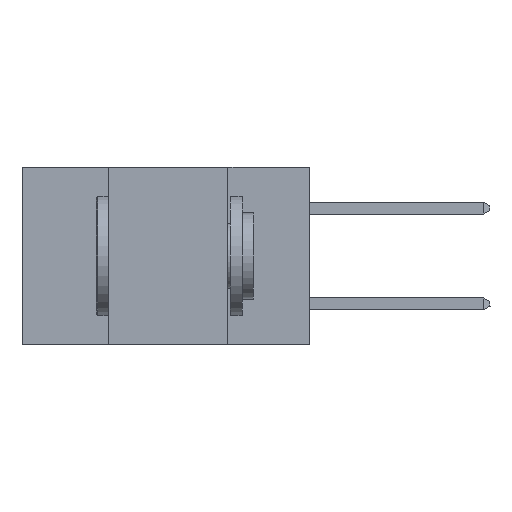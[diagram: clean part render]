
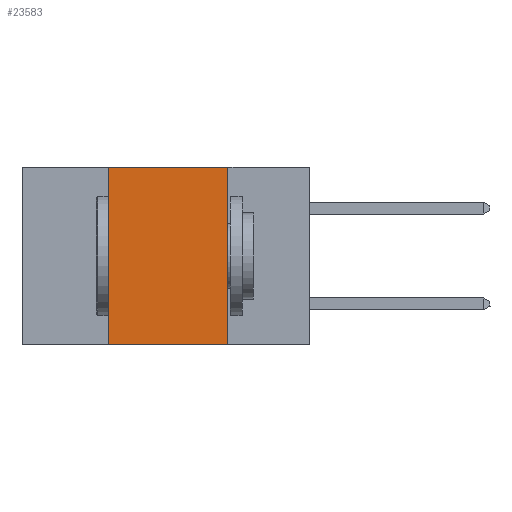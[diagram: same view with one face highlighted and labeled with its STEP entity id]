
A CAD part, left-side view. The second image highlights one B-rep face of the part: STEP entity #23583.
In plain terms, the highlighted planar face has unit normal (-1, 0, 0).
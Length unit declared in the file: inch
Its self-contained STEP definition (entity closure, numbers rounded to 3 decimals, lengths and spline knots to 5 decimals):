
#287 = DIRECTION ( 'NONE',  ( 0., 0., -1. ) ) ;
#386 = EDGE_CURVE ( 'NONE', #21851, #12763, #11255, .T. ) ;
#1092 = CARTESIAN_POINT ( 'NONE',  ( 0., 0.6, -0.37 ) ) ;
#1902 = VERTEX_POINT ( 'NONE', #4614 ) ;
#2606 = PLANE ( 'NONE',  #6581 ) ;
#4350 = LINE ( 'NONE', #14919, #22343 ) ;
#4395 = VECTOR ( 'NONE', #7131, 39.37008 ) ;
#4614 = CARTESIAN_POINT ( 'NONE',  ( 0., 0.42, 0. ) ) ;
#6141 = VECTOR ( 'NONE', #23183, 39.37008 ) ;
#6581 = AXIS2_PLACEMENT_3D ( 'NONE', #12124, #24663, #287 ) ;
#7131 = DIRECTION ( 'NONE',  ( 0., 0., -1. ) ) ;
#8068 = EDGE_CURVE ( 'NONE', #1902, #21851, #17598, .T. ) ;
#11255 = LINE ( 'NONE', #24590, #4395 ) ;
#11903 = CARTESIAN_POINT ( 'NONE',  ( 0., 0.17, -0.37 ) ) ;
#12083 = EDGE_LOOP ( 'NONE', ( #14166, #24824, #24048, #15727 ) ) ;
#12124 = CARTESIAN_POINT ( 'NONE',  ( 0., 0.6, 0. ) ) ;
#12763 = VERTEX_POINT ( 'NONE', #11903 ) ;
#14166 = ORIENTED_EDGE ( 'NONE', *, *, #386, .F. ) ;
#14205 = CARTESIAN_POINT ( 'NONE',  ( 0., 0.17, 0. ) ) ;
#14919 = CARTESIAN_POINT ( 'NONE',  ( 0., 0.42, 0. ) ) ;
#15727 = ORIENTED_EDGE ( 'NONE', *, *, #16045, .T. ) ;
#16045 = EDGE_CURVE ( 'NONE', #31651, #12763, #21640, .T. ) ;
#17598 = LINE ( 'NONE', #25449, #6141 ) ;
#18444 = DIRECTION ( 'NONE',  ( 0., -1., 0. ) ) ;
#19997 = DIRECTION ( 'NONE',  ( 0., 0., 1. ) ) ;
#20476 = VECTOR ( 'NONE', #18444, 39.37008 ) ;
#21640 = LINE ( 'NONE', #1092, #20476 ) ;
#21851 = VERTEX_POINT ( 'NONE', #14205 ) ;
#22343 = VECTOR ( 'NONE', #19997, 39.37008 ) ;
#23183 = DIRECTION ( 'NONE',  ( 0., -1., 0. ) ) ;
#23583 = ADVANCED_FACE ( 'NONE', ( #25181 ), #2606, .F. ) ;
#24048 = ORIENTED_EDGE ( 'NONE', *, *, #26654, .F. ) ;
#24590 = CARTESIAN_POINT ( 'NONE',  ( 0., 0.17, 0. ) ) ;
#24663 = DIRECTION ( 'NONE',  ( 1., 0., 0. ) ) ;
#24824 = ORIENTED_EDGE ( 'NONE', *, *, #8068, .F. ) ;
#25181 = FACE_OUTER_BOUND ( 'NONE', #12083, .T. ) ;
#25449 = CARTESIAN_POINT ( 'NONE',  ( 0., 0.6, 0. ) ) ;
#26654 = EDGE_CURVE ( 'NONE', #31651, #1902, #4350, .T. ) ;
#27302 = CARTESIAN_POINT ( 'NONE',  ( 0., 0.42, -0.37 ) ) ;
#31651 = VERTEX_POINT ( 'NONE', #27302 ) ;
